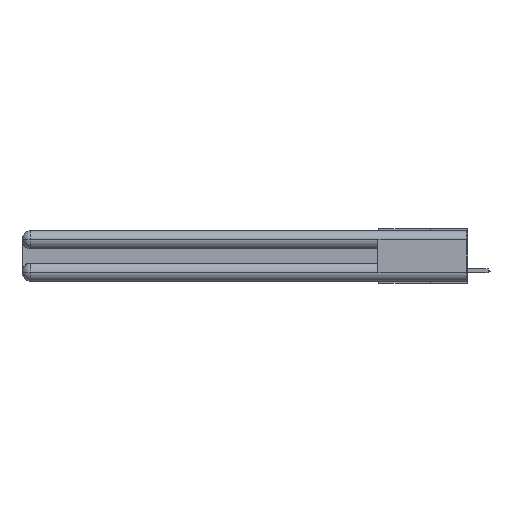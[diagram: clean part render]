
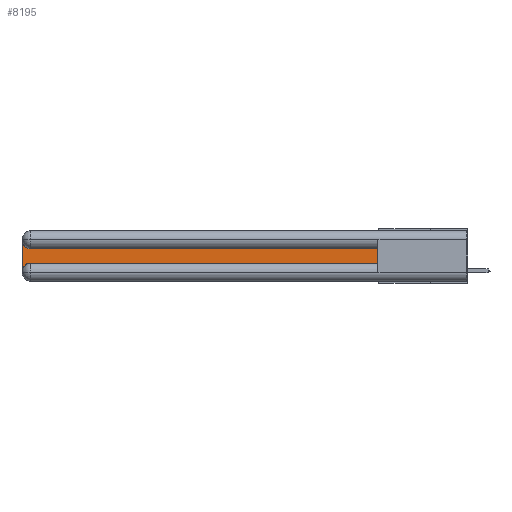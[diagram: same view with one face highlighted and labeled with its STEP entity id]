
A CAD part, left-side view. The second image highlights one B-rep face of the part: STEP entity #8195.
In plain terms, the highlighted planar face has unit normal (-1, 0, 0).
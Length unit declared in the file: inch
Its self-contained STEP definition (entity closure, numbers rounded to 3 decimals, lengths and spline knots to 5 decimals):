
#256 = DIRECTION ( 'NONE',  ( 0., 0., -1. ) ) ;
#790 = EDGE_CURVE ( 'NONE', #5519, #23109, #19278, .T. ) ;
#882 = VERTEX_POINT ( 'NONE', #29754 ) ;
#1592 = DIRECTION ( 'NONE',  ( 0., 0., 1. ) ) ;
#2339 = CARTESIAN_POINT ( 'NONE',  ( 0.075, 2.94, -0.2775 ) ) ;
#2546 = DIRECTION ( 'NONE',  ( 1., 0., 0. ) ) ;
#2784 = DIRECTION ( 'NONE',  ( 0., 0., -1. ) ) ;
#3520 = EDGE_CURVE ( 'NONE', #23109, #882, #30760, .T. ) ;
#3955 = EDGE_CURVE ( 'NONE', #25633, #28489, #11128, .T. ) ;
#5519 = VERTEX_POINT ( 'NONE', #26760 ) ;
#6121 = EDGE_CURVE ( 'NONE', #7258, #25633, #6492, .T. ) ;
#6492 = CIRCLE ( 'NONE', #7412, 0.06 ) ;
#6647 = DIRECTION ( 'NONE',  ( 0., 0., -1. ) ) ;
#7258 = VERTEX_POINT ( 'NONE', #12284 ) ;
#7412 = AXIS2_PLACEMENT_3D ( 'NONE', #13943, #11803, #6647 ) ;
#7728 = CARTESIAN_POINT ( 'NONE',  ( 0.075, 0.6, -0.2175 ) ) ;
#7741 = FACE_OUTER_BOUND ( 'NONE', #18807, .T. ) ;
#8195 = ADVANCED_FACE ( 'NONE', ( #7741 ), #11778, .F. ) ;
#8418 = CARTESIAN_POINT ( 'NONE',  ( 0.075, 0.6, -0.1225 ) ) ;
#9499 = ORIENTED_EDGE ( 'NONE', *, *, #3955, .T. ) ;
#10419 = VECTOR ( 'NONE', #17856, 39.37008 ) ;
#10649 = ORIENTED_EDGE ( 'NONE', *, *, #6121, .T. ) ;
#11128 = LINE ( 'NONE', #12428, #28663 ) ;
#11317 = VECTOR ( 'NONE', #1592, 39.37008 ) ;
#11778 = PLANE ( 'NONE',  #29216 ) ;
#11803 = DIRECTION ( 'NONE',  ( 1., 0., 0. ) ) ;
#12284 = CARTESIAN_POINT ( 'NONE',  ( 0.075, 2.94, -0.1225 ) ) ;
#12428 = CARTESIAN_POINT ( 'NONE',  ( 0.075, 3., -0.2175 ) ) ;
#12787 = ORIENTED_EDGE ( 'NONE', *, *, #22562, .T. ) ;
#13877 = ORIENTED_EDGE ( 'NONE', *, *, #18032, .T. ) ;
#13943 = CARTESIAN_POINT ( 'NONE',  ( 0.075, 2.94, -0.0625 ) ) ;
#15184 = AXIS2_PLACEMENT_3D ( 'NONE', #2339, #2546, #256 ) ;
#15228 = ORIENTED_EDGE ( 'NONE', *, *, #3520, .T. ) ;
#16035 = DIRECTION ( 'NONE',  ( 0., -1., 0. ) ) ;
#16874 = DIRECTION ( 'NONE',  ( 1., 0., 0. ) ) ;
#17268 = CARTESIAN_POINT ( 'NONE',  ( 0.075, 3., -0.0625 ) ) ;
#17856 = DIRECTION ( 'NONE',  ( 0., 1., 0. ) ) ;
#18032 = EDGE_CURVE ( 'NONE', #882, #7258, #28688, .T. ) ;
#18807 = EDGE_LOOP ( 'NONE', ( #13877, #10649, #9499, #12787, #29515, #15228 ) ) ;
#19278 = LINE ( 'NONE', #28173, #23121 ) ;
#21557 = CARTESIAN_POINT ( 'NONE',  ( 0.075, 3., -0.1225 ) ) ;
#21783 = DIRECTION ( 'NONE',  ( 0., 0., -1. ) ) ;
#22562 = EDGE_CURVE ( 'NONE', #28489, #5519, #26351, .T. ) ;
#23109 = VERTEX_POINT ( 'NONE', #7728 ) ;
#23121 = VECTOR ( 'NONE', #16035, 39.37008 ) ;
#25633 = VERTEX_POINT ( 'NONE', #17268 ) ;
#26351 = CIRCLE ( 'NONE', #15184, 0.06 ) ;
#26760 = CARTESIAN_POINT ( 'NONE',  ( 0.075, 2.94, -0.2175 ) ) ;
#28173 = CARTESIAN_POINT ( 'NONE',  ( 0.075, 0.6, -0.2175 ) ) ;
#28182 = CARTESIAN_POINT ( 'NONE',  ( 0.075, 3., -0.2775 ) ) ;
#28437 = CARTESIAN_POINT ( 'NONE',  ( 0.075, 0.6, -0.2175 ) ) ;
#28489 = VERTEX_POINT ( 'NONE', #28182 ) ;
#28663 = VECTOR ( 'NONE', #2784, 39.37008 ) ;
#28688 = LINE ( 'NONE', #8418, #10419 ) ;
#29216 = AXIS2_PLACEMENT_3D ( 'NONE', #21557, #16874, #21783 ) ;
#29515 = ORIENTED_EDGE ( 'NONE', *, *, #790, .T. ) ;
#29754 = CARTESIAN_POINT ( 'NONE',  ( 0.075, 0.6, -0.1225 ) ) ;
#30760 = LINE ( 'NONE', #28437, #11317 ) ;
